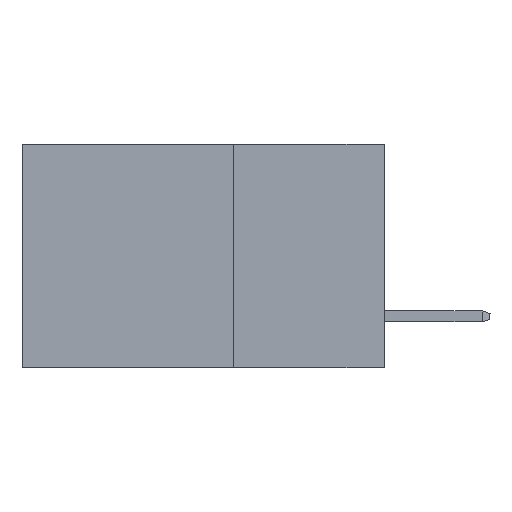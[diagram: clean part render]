
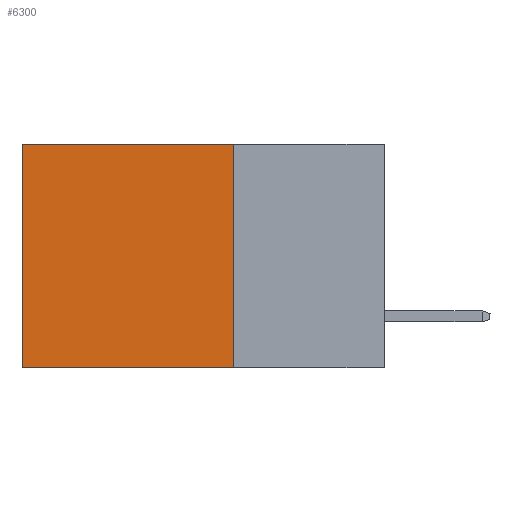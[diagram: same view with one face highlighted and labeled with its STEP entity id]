
A CAD part, left-side view. The second image highlights one B-rep face of the part: STEP entity #6300.
In plain terms, the highlighted planar face has unit normal (-1, 0, 0).
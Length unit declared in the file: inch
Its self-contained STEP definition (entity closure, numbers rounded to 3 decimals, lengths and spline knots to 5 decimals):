
#259 = LINE ( 'NONE', #8889, #7917 ) ;
#396 = DIRECTION ( 'NONE',  ( 0., 1., 0. ) ) ;
#803 = VERTEX_POINT ( 'NONE', #11526 ) ;
#1026 = FACE_OUTER_BOUND ( 'NONE', #5301, .T. ) ;
#1129 = VECTOR ( 'NONE', #6370, 39.37008 ) ;
#1348 = EDGE_CURVE ( 'NONE', #803, #7536, #2313, .T. ) ;
#1927 = ORIENTED_EDGE ( 'NONE', *, *, #5227, .T. ) ;
#2313 = LINE ( 'NONE', #3070, #8691 ) ;
#2316 = CARTESIAN_POINT ( 'NONE',  ( 0.2615, 0.6, -0.37 ) ) ;
#2546 = LINE ( 'NONE', #9251, #4752 ) ;
#3006 = DIRECTION ( 'NONE',  ( 1., 0., 0. ) ) ;
#3012 = CARTESIAN_POINT ( 'NONE',  ( 0.2615, 0.6, 0. ) ) ;
#3070 = CARTESIAN_POINT ( 'NONE',  ( 0.2615, 0.25, -0.37 ) ) ;
#3231 = ORIENTED_EDGE ( 'NONE', *, *, #1348, .F. ) ;
#3604 = VERTEX_POINT ( 'NONE', #3012 ) ;
#3821 = PLANE ( 'NONE',  #10116 ) ;
#4253 = EDGE_CURVE ( 'NONE', #4566, #803, #259, .T. ) ;
#4414 = EDGE_CURVE ( 'NONE', #4566, #3604, #2546, .T. ) ;
#4566 = VERTEX_POINT ( 'NONE', #5598 ) ;
#4752 = VECTOR ( 'NONE', #11924, 39.37008 ) ;
#5227 = EDGE_CURVE ( 'NONE', #3604, #7536, #8228, .T. ) ;
#5301 = EDGE_LOOP ( 'NONE', ( #1927, #3231, #12015, #5559 ) ) ;
#5559 = ORIENTED_EDGE ( 'NONE', *, *, #4414, .T. ) ;
#5598 = CARTESIAN_POINT ( 'NONE',  ( 0.2615, 0.25, 0. ) ) ;
#6300 = ADVANCED_FACE ( 'NONE', ( #1026 ), #3821, .F. ) ;
#6370 = DIRECTION ( 'NONE',  ( 0., 0., -1. ) ) ;
#7536 = VERTEX_POINT ( 'NONE', #2316 ) ;
#7864 = DIRECTION ( 'NONE',  ( 0., 0., -1. ) ) ;
#7917 = VECTOR ( 'NONE', #9939, 39.37008 ) ;
#8167 = CARTESIAN_POINT ( 'NONE',  ( 0.2615, 0.6, -0.37 ) ) ;
#8228 = LINE ( 'NONE', #8167, #1129 ) ;
#8603 = CARTESIAN_POINT ( 'NONE',  ( 0.2615, 0.25, -0.37 ) ) ;
#8691 = VECTOR ( 'NONE', #396, 39.37008 ) ;
#8889 = CARTESIAN_POINT ( 'NONE',  ( 0.2615, 0.25, -0.37 ) ) ;
#9251 = CARTESIAN_POINT ( 'NONE',  ( 0.2615, 0.25, 0. ) ) ;
#9939 = DIRECTION ( 'NONE',  ( 0., 0., -1. ) ) ;
#10116 = AXIS2_PLACEMENT_3D ( 'NONE', #8603, #3006, #7864 ) ;
#11526 = CARTESIAN_POINT ( 'NONE',  ( 0.2615, 0.25, -0.37 ) ) ;
#11924 = DIRECTION ( 'NONE',  ( 0., 1., 0. ) ) ;
#12015 = ORIENTED_EDGE ( 'NONE', *, *, #4253, .F. ) ;
